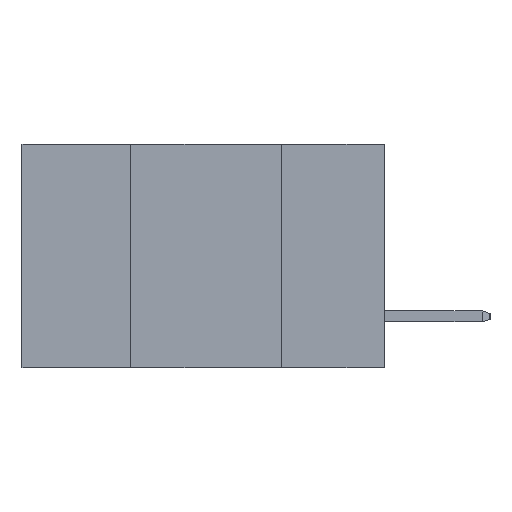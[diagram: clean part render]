
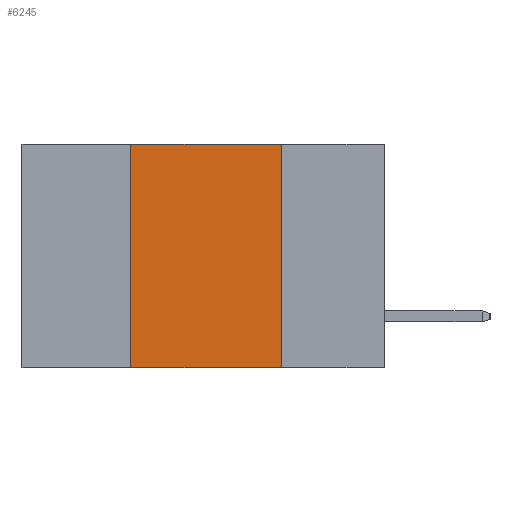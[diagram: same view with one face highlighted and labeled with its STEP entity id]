
A CAD part, left-side view. The second image highlights one B-rep face of the part: STEP entity #6245.
In plain terms, the highlighted planar face has unit normal (-1, 0, 0).
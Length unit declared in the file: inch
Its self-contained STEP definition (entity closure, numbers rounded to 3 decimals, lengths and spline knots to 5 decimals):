
#950 = DIRECTION ( 'NONE',  ( 0., -1., 0. ) ) ;
#1244 = CARTESIAN_POINT ( 'NONE',  ( 0., 0.6, 0. ) ) ;
#1287 = VERTEX_POINT ( 'NONE', #19643 ) ;
#1309 = EDGE_CURVE ( 'NONE', #11950, #19236, #16166, .T. ) ;
#1816 = VECTOR ( 'NONE', #950, 39.37008 ) ;
#2749 = LINE ( 'NONE', #9758, #6895 ) ;
#2830 = DIRECTION ( 'NONE',  ( 0., 0., -1. ) ) ;
#3462 = EDGE_LOOP ( 'NONE', ( #15013, #15487, #19444, #4299 ) ) ;
#3527 = LINE ( 'NONE', #15185, #11259 ) ;
#4299 = ORIENTED_EDGE ( 'NONE', *, *, #17074, .T. ) ;
#4518 = VECTOR ( 'NONE', #19452, 39.37008 ) ;
#5661 = EDGE_CURVE ( 'NONE', #6512, #11950, #18049, .T. ) ;
#6245 = ADVANCED_FACE ( 'NONE', ( #11951 ), #7790, .F. ) ;
#6510 = EDGE_CURVE ( 'NONE', #1287, #6512, #3527, .T. ) ;
#6512 = VERTEX_POINT ( 'NONE', #15250 ) ;
#6895 = VECTOR ( 'NONE', #11232, 39.37008 ) ;
#7790 = PLANE ( 'NONE',  #10860 ) ;
#8477 = CARTESIAN_POINT ( 'NONE',  ( 0., 0.17, 0. ) ) ;
#9758 = CARTESIAN_POINT ( 'NONE',  ( 0., 0.6, -0.37 ) ) ;
#10519 = DIRECTION ( 'NONE',  ( 1., 0., 0. ) ) ;
#10860 = AXIS2_PLACEMENT_3D ( 'NONE', #10929, #10519, #2830 ) ;
#10929 = CARTESIAN_POINT ( 'NONE',  ( 0., 0.6, 0. ) ) ;
#11232 = DIRECTION ( 'NONE',  ( 0., -1., 0. ) ) ;
#11259 = VECTOR ( 'NONE', #14124, 39.37008 ) ;
#11540 = CARTESIAN_POINT ( 'NONE',  ( 0., 0.17, -0.37 ) ) ;
#11950 = VERTEX_POINT ( 'NONE', #8477 ) ;
#11951 = FACE_OUTER_BOUND ( 'NONE', #3462, .T. ) ;
#14124 = DIRECTION ( 'NONE',  ( 0., 0., 1. ) ) ;
#15013 = ORIENTED_EDGE ( 'NONE', *, *, #1309, .F. ) ;
#15185 = CARTESIAN_POINT ( 'NONE',  ( 0., 0.42, 0. ) ) ;
#15250 = CARTESIAN_POINT ( 'NONE',  ( 0., 0.42, 0. ) ) ;
#15487 = ORIENTED_EDGE ( 'NONE', *, *, #5661, .F. ) ;
#16166 = LINE ( 'NONE', #16552, #4518 ) ;
#16552 = CARTESIAN_POINT ( 'NONE',  ( 0., 0.17, 0. ) ) ;
#17074 = EDGE_CURVE ( 'NONE', #1287, #19236, #2749, .T. ) ;
#18049 = LINE ( 'NONE', #1244, #1816 ) ;
#19236 = VERTEX_POINT ( 'NONE', #11540 ) ;
#19444 = ORIENTED_EDGE ( 'NONE', *, *, #6510, .F. ) ;
#19452 = DIRECTION ( 'NONE',  ( 0., 0., -1. ) ) ;
#19643 = CARTESIAN_POINT ( 'NONE',  ( 0., 0.42, -0.37 ) ) ;
